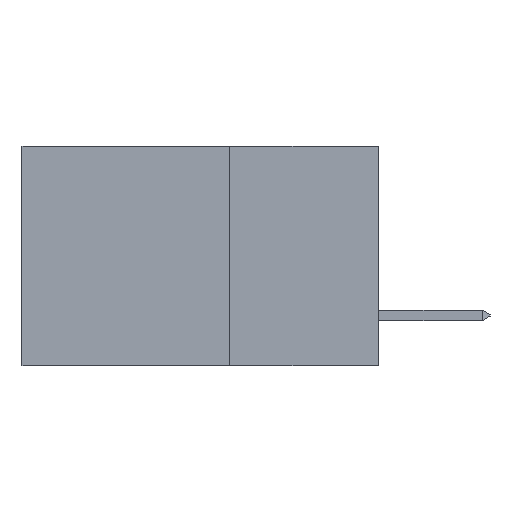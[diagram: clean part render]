
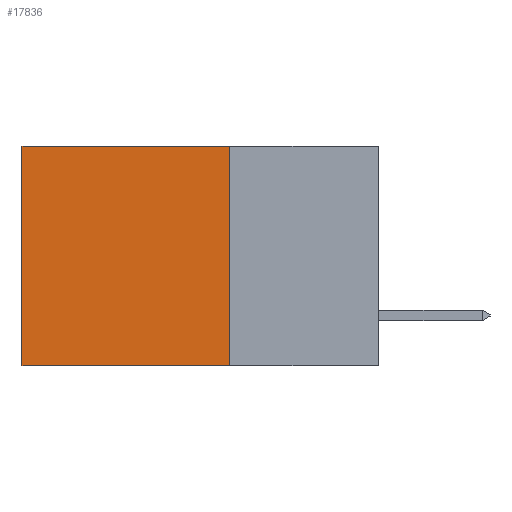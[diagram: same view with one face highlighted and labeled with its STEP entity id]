
A CAD part, left-side view. The second image highlights one B-rep face of the part: STEP entity #17836.
In plain terms, the highlighted planar face has unit normal (-1, 0, 0).
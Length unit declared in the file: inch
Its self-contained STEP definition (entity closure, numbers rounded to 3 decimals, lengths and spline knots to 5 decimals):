
#676 = LINE ( 'NONE', #19925, #13111 ) ;
#1318 = VECTOR ( 'NONE', #10776, 39.37008 ) ;
#1580 = VERTEX_POINT ( 'NONE', #12184 ) ;
#1597 = CARTESIAN_POINT ( 'NONE',  ( 0.298, 0.25, 0. ) ) ;
#2277 = DIRECTION ( 'NONE',  ( 0., 0., -1. ) ) ;
#2313 = FACE_OUTER_BOUND ( 'NONE', #15470, .T. ) ;
#2482 = ORIENTED_EDGE ( 'NONE', *, *, #10050, .F. ) ;
#2997 = EDGE_CURVE ( 'NONE', #17819, #1580, #17167, .T. ) ;
#3186 = ORIENTED_EDGE ( 'NONE', *, *, #12982, .T. ) ;
#4768 = DIRECTION ( 'NONE',  ( 0., 0., -1. ) ) ;
#4832 = VECTOR ( 'NONE', #11381, 39.37008 ) ;
#4908 = DIRECTION ( 'NONE',  ( 0., 0., -1. ) ) ;
#7575 = CARTESIAN_POINT ( 'NONE',  ( 0.298, 0.6, 0. ) ) ;
#7758 = CARTESIAN_POINT ( 'NONE',  ( 0.298, 0.25, 0. ) ) ;
#9506 = AXIS2_PLACEMENT_3D ( 'NONE', #1597, #14601, #4908 ) ;
#9856 = VERTEX_POINT ( 'NONE', #7575 ) ;
#9983 = LINE ( 'NONE', #18739, #1318 ) ;
#10050 = EDGE_CURVE ( 'NONE', #20418, #17819, #12256, .T. ) ;
#10424 = CARTESIAN_POINT ( 'NONE',  ( 0.298, 0.25, -0.37 ) ) ;
#10776 = DIRECTION ( 'NONE',  ( 0., 1., 0. ) ) ;
#11329 = PLANE ( 'NONE',  #9506 ) ;
#11381 = DIRECTION ( 'NONE',  ( 0., 1., 0. ) ) ;
#12184 = CARTESIAN_POINT ( 'NONE',  ( 0.298, 0.6, -0.37 ) ) ;
#12256 = LINE ( 'NONE', #19232, #20711 ) ;
#12982 = EDGE_CURVE ( 'NONE', #9856, #1580, #676, .T. ) ;
#13111 = VECTOR ( 'NONE', #2277, 39.37008 ) ;
#14178 = ORIENTED_EDGE ( 'NONE', *, *, #16659, .T. ) ;
#14601 = DIRECTION ( 'NONE',  ( 1., 0., 0. ) ) ;
#15470 = EDGE_LOOP ( 'NONE', ( #3186, #19858, #2482, #14178 ) ) ;
#16659 = EDGE_CURVE ( 'NONE', #20418, #9856, #9983, .T. ) ;
#17167 = LINE ( 'NONE', #10424, #4832 ) ;
#17819 = VERTEX_POINT ( 'NONE', #20808 ) ;
#17836 = ADVANCED_FACE ( 'NONE', ( #2313 ), #11329, .F. ) ;
#18739 = CARTESIAN_POINT ( 'NONE',  ( 0.298, 0.25, 0. ) ) ;
#19232 = CARTESIAN_POINT ( 'NONE',  ( 0.298, 0.25, 0. ) ) ;
#19858 = ORIENTED_EDGE ( 'NONE', *, *, #2997, .F. ) ;
#19925 = CARTESIAN_POINT ( 'NONE',  ( 0.298, 0.6, 0. ) ) ;
#20418 = VERTEX_POINT ( 'NONE', #7758 ) ;
#20711 = VECTOR ( 'NONE', #4768, 39.37008 ) ;
#20808 = CARTESIAN_POINT ( 'NONE',  ( 0.298, 0.25, -0.37 ) ) ;
